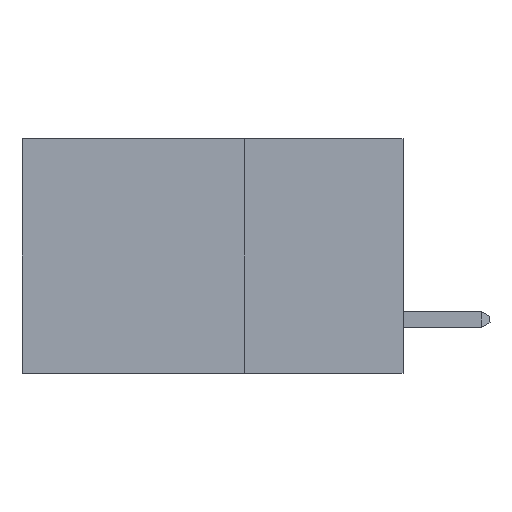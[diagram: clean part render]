
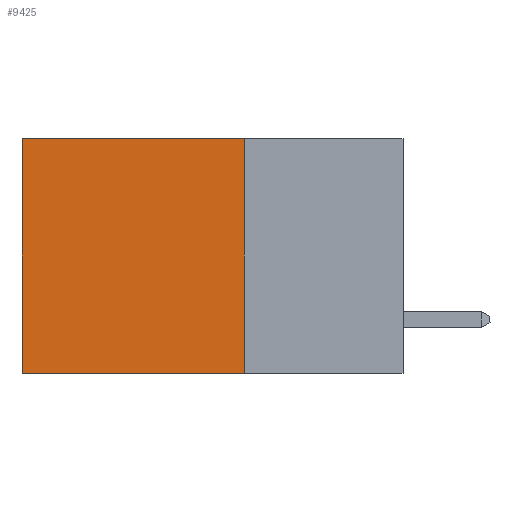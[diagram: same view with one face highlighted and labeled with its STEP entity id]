
A CAD part, left-side view. The second image highlights one B-rep face of the part: STEP entity #9425.
In plain terms, the highlighted planar face has unit normal (-1, 0, 0).
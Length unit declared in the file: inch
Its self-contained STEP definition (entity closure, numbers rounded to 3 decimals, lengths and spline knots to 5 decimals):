
#136 = CARTESIAN_POINT ( 'NONE',  ( 0.2875, 0.6, -0.37 ) ) ;
#163 = LINE ( 'NONE', #19314, #4468 ) ;
#855 = VECTOR ( 'NONE', #18820, 39.37008 ) ;
#1194 = ORIENTED_EDGE ( 'NONE', *, *, #9983, .F. ) ;
#1332 = LINE ( 'NONE', #11195, #855 ) ;
#1570 = AXIS2_PLACEMENT_3D ( 'NONE', #6294, #18892, #9452 ) ;
#1582 = CARTESIAN_POINT ( 'NONE',  ( 0.2875, 0.25, -0.37 ) ) ;
#1728 = DIRECTION ( 'NONE',  ( 0., 1., 0. ) ) ;
#1854 = EDGE_CURVE ( 'NONE', #14432, #6476, #1332, .T. ) ;
#2534 = VECTOR ( 'NONE', #2576, 39.37008 ) ;
#2576 = DIRECTION ( 'NONE',  ( 0., 1., 0. ) ) ;
#3069 = VERTEX_POINT ( 'NONE', #1582 ) ;
#3124 = PLANE ( 'NONE',  #1570 ) ;
#3200 = ORIENTED_EDGE ( 'NONE', *, *, #15006, .T. ) ;
#4468 = VECTOR ( 'NONE', #11427, 39.37008 ) ;
#4953 = VERTEX_POINT ( 'NONE', #20026 ) ;
#5762 = VECTOR ( 'NONE', #1728, 39.37008 ) ;
#6294 = CARTESIAN_POINT ( 'NONE',  ( 0.2875, 0.25, 0. ) ) ;
#6455 = ORIENTED_EDGE ( 'NONE', *, *, #11669, .F. ) ;
#6476 = VERTEX_POINT ( 'NONE', #136 ) ;
#9425 = ADVANCED_FACE ( 'NONE', ( #11639 ), #3124, .F. ) ;
#9452 = DIRECTION ( 'NONE',  ( 0., 0., -1. ) ) ;
#9983 = EDGE_CURVE ( 'NONE', #3069, #6476, #14040, .T. ) ;
#10320 = CARTESIAN_POINT ( 'NONE',  ( 0.2875, 0.6, 0. ) ) ;
#11195 = CARTESIAN_POINT ( 'NONE',  ( 0.2875, 0.6, 0. ) ) ;
#11427 = DIRECTION ( 'NONE',  ( 0., 0., -1. ) ) ;
#11626 = ORIENTED_EDGE ( 'NONE', *, *, #1854, .T. ) ;
#11639 = FACE_OUTER_BOUND ( 'NONE', #12501, .T. ) ;
#11669 = EDGE_CURVE ( 'NONE', #4953, #3069, #163, .T. ) ;
#11986 = CARTESIAN_POINT ( 'NONE',  ( 0.2875, 0.25, 0. ) ) ;
#12501 = EDGE_LOOP ( 'NONE', ( #11626, #1194, #6455, #3200 ) ) ;
#14040 = LINE ( 'NONE', #19071, #5762 ) ;
#14432 = VERTEX_POINT ( 'NONE', #10320 ) ;
#15006 = EDGE_CURVE ( 'NONE', #4953, #14432, #19301, .T. ) ;
#18820 = DIRECTION ( 'NONE',  ( 0., 0., -1. ) ) ;
#18892 = DIRECTION ( 'NONE',  ( 1., 0., 0. ) ) ;
#19071 = CARTESIAN_POINT ( 'NONE',  ( 0.2875, 0.25, -0.37 ) ) ;
#19301 = LINE ( 'NONE', #11986, #2534 ) ;
#19314 = CARTESIAN_POINT ( 'NONE',  ( 0.2875, 0.25, 0. ) ) ;
#20026 = CARTESIAN_POINT ( 'NONE',  ( 0.2875, 0.25, 0. ) ) ;
